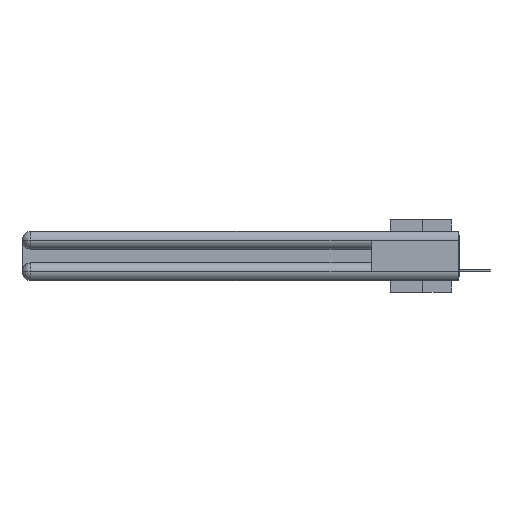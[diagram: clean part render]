
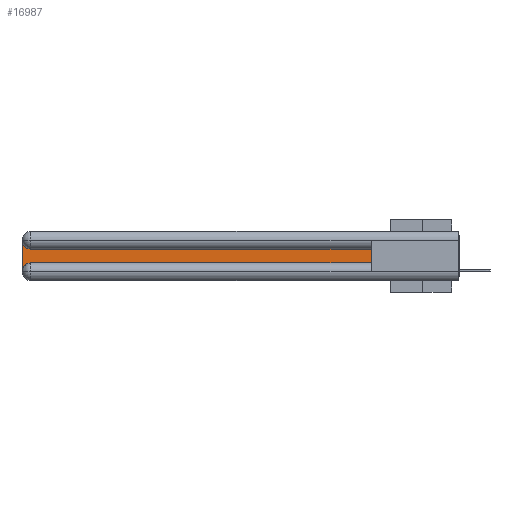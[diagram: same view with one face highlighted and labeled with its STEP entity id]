
A CAD part, left-side view. The second image highlights one B-rep face of the part: STEP entity #16987.
In plain terms, the highlighted planar face has unit normal (-1, 0, 0).
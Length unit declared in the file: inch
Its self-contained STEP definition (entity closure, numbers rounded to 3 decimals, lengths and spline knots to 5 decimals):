
#351 = DIRECTION ( 'NONE',  ( 0., 0., -1. ) ) ;
#450 = CARTESIAN_POINT ( 'NONE',  ( 0.075, 0.6, -0.2175 ) ) ;
#1077 = EDGE_LOOP ( 'NONE', ( #23945, #28196, #11532, #4526, #19036, #4729 ) ) ;
#1536 = VERTEX_POINT ( 'NONE', #19642 ) ;
#3214 = DIRECTION ( 'NONE',  ( 1., 0., 0. ) ) ;
#4355 = VERTEX_POINT ( 'NONE', #20430 ) ;
#4526 = ORIENTED_EDGE ( 'NONE', *, *, #21613, .T. ) ;
#4729 = ORIENTED_EDGE ( 'NONE', *, *, #19245, .T. ) ;
#4999 = DIRECTION ( 'NONE',  ( 0., 0., -1. ) ) ;
#5551 = CARTESIAN_POINT ( 'NONE',  ( 0.075, 2.94, -0.2775 ) ) ;
#6354 = DIRECTION ( 'NONE',  ( 0., -1., 0. ) ) ;
#6436 = DIRECTION ( 'NONE',  ( 1., 0., 0. ) ) ;
#7639 = VERTEX_POINT ( 'NONE', #29932 ) ;
#7989 = CARTESIAN_POINT ( 'NONE',  ( 0.075, 0.6, -0.1225 ) ) ;
#8089 = AXIS2_PLACEMENT_3D ( 'NONE', #23664, #6436, #18743 ) ;
#8929 = LINE ( 'NONE', #22984, #25542 ) ;
#9566 = VECTOR ( 'NONE', #6354, 39.37008 ) ;
#9690 = EDGE_CURVE ( 'NONE', #17086, #19239, #25431, .T. ) ;
#9898 = FACE_OUTER_BOUND ( 'NONE', #1077, .T. ) ;
#11532 = ORIENTED_EDGE ( 'NONE', *, *, #13096, .T. ) ;
#12360 = CARTESIAN_POINT ( 'NONE',  ( 0.075, 3., -0.2775 ) ) ;
#13036 = PLANE ( 'NONE',  #32416 ) ;
#13096 = EDGE_CURVE ( 'NONE', #1536, #14871, #28286, .T. ) ;
#13551 = LINE ( 'NONE', #450, #9566 ) ;
#14871 = VERTEX_POINT ( 'NONE', #12360 ) ;
#15605 = DIRECTION ( 'NONE',  ( 1., 0., 0. ) ) ;
#16072 = DIRECTION ( 'NONE',  ( 0., 1., 0. ) ) ;
#16878 = CARTESIAN_POINT ( 'NONE',  ( 0.075, 0.6, -0.1225 ) ) ;
#16987 = ADVANCED_FACE ( 'NONE', ( #9898 ), #13036, .F. ) ;
#17086 = VERTEX_POINT ( 'NONE', #7989 ) ;
#17468 = AXIS2_PLACEMENT_3D ( 'NONE', #5551, #15605, #351 ) ;
#17967 = CARTESIAN_POINT ( 'NONE',  ( 0.075, 2.94, -0.1225 ) ) ;
#18061 = VECTOR ( 'NONE', #25874, 39.37008 ) ;
#18514 = CARTESIAN_POINT ( 'NONE',  ( 0.075, 3., -0.2175 ) ) ;
#18743 = DIRECTION ( 'NONE',  ( 0., 0., -1. ) ) ;
#19036 = ORIENTED_EDGE ( 'NONE', *, *, #20078, .T. ) ;
#19239 = VERTEX_POINT ( 'NONE', #17967 ) ;
#19245 = EDGE_CURVE ( 'NONE', #7639, #17086, #8929, .T. ) ;
#19642 = CARTESIAN_POINT ( 'NONE',  ( 0.075, 3., -0.0625 ) ) ;
#20078 = EDGE_CURVE ( 'NONE', #4355, #7639, #13551, .T. ) ;
#20430 = CARTESIAN_POINT ( 'NONE',  ( 0.075, 2.94, -0.2175 ) ) ;
#21613 = EDGE_CURVE ( 'NONE', #14871, #4355, #26862, .T. ) ;
#22514 = EDGE_CURVE ( 'NONE', #19239, #1536, #31522, .T. ) ;
#22984 = CARTESIAN_POINT ( 'NONE',  ( 0.075, 0.6, -0.2175 ) ) ;
#23664 = CARTESIAN_POINT ( 'NONE',  ( 0.075, 2.94, -0.0625 ) ) ;
#23945 = ORIENTED_EDGE ( 'NONE', *, *, #9690, .T. ) ;
#25431 = LINE ( 'NONE', #16878, #32200 ) ;
#25542 = VECTOR ( 'NONE', #30526, 39.37008 ) ;
#25874 = DIRECTION ( 'NONE',  ( 0., 0., -1. ) ) ;
#26862 = CIRCLE ( 'NONE', #17468, 0.06 ) ;
#28196 = ORIENTED_EDGE ( 'NONE', *, *, #22514, .T. ) ;
#28286 = LINE ( 'NONE', #18514, #18061 ) ;
#29932 = CARTESIAN_POINT ( 'NONE',  ( 0.075, 0.6, -0.2175 ) ) ;
#30526 = DIRECTION ( 'NONE',  ( 0., 0., 1. ) ) ;
#30704 = CARTESIAN_POINT ( 'NONE',  ( 0.075, 3., -0.1225 ) ) ;
#31522 = CIRCLE ( 'NONE', #8089, 0.06 ) ;
#32200 = VECTOR ( 'NONE', #16072, 39.37008 ) ;
#32416 = AXIS2_PLACEMENT_3D ( 'NONE', #30704, #3214, #4999 ) ;
